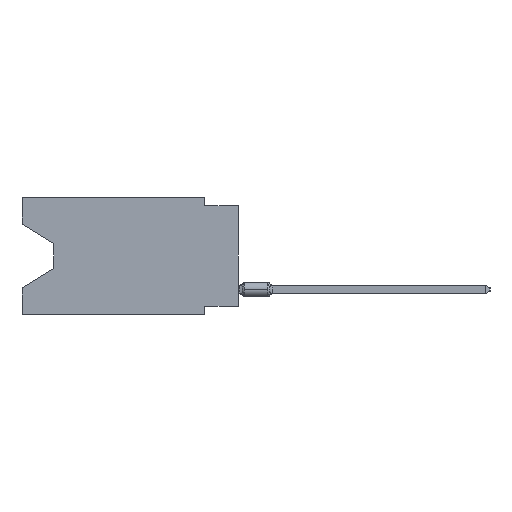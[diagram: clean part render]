
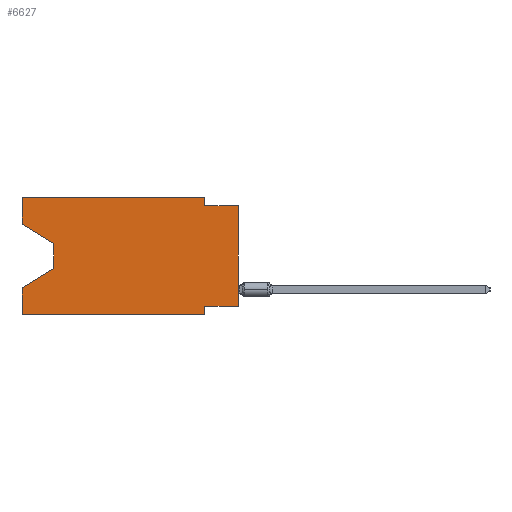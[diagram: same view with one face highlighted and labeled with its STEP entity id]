
A CAD part, left-side view. The second image highlights one B-rep face of the part: STEP entity #6627.
In plain terms, the highlighted planar face has unit normal (-1, 0, 0).
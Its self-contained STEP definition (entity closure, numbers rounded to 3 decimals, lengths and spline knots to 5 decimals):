
#2103 = ORIENTED_EDGE ( 'NONE', *, *, #78197, .T. ) ;
#3496 = DIRECTION ( 'NONE',  ( 1., 0., 0. ) ) ;
#4381 = CARTESIAN_POINT ( 'NONE',  ( 0., 0.645, -0.35 ) ) ;
#5748 = VERTEX_POINT ( 'NONE', #39339 ) ;
#6627 = ADVANCED_FACE ( 'NONE', ( #53965 ), #81701, .F. ) ;
#6694 = CARTESIAN_POINT ( 'NONE',  ( 0., 0.645, -0.08025 ) ) ;
#7017 = LINE ( 'NONE', #53171, #76037 ) ;
#8614 = LINE ( 'NONE', #80415, #32343 ) ;
#9601 = CARTESIAN_POINT ( 'NONE',  ( 0., 0.1, -0.35 ) ) ;
#10518 = LINE ( 'NONE', #36602, #60691 ) ;
#10760 = LINE ( 'NONE', #16331, #52014 ) ;
#13419 = DIRECTION ( 'NONE',  ( 0., -1., 0. ) ) ;
#14014 = CARTESIAN_POINT ( 'NONE',  ( 0., 0.1, -0.025 ) ) ;
#14071 = VERTEX_POINT ( 'NONE', #52846 ) ;
#14917 = ORIENTED_EDGE ( 'NONE', *, *, #15373, .T. ) ;
#15373 = EDGE_CURVE ( 'NONE', #57715, #5748, #27320, .T. ) ;
#16026 = ORIENTED_EDGE ( 'NONE', *, *, #21069, .F. ) ;
#16331 = CARTESIAN_POINT ( 'NONE',  ( 0., 0.645, -0.35 ) ) ;
#17406 = DIRECTION ( 'NONE',  ( 0., -1., 0. ) ) ;
#17515 = CARTESIAN_POINT ( 'NONE',  ( 0., 0.1, -0.325 ) ) ;
#19290 = VECTOR ( 'NONE', #52750, 39.37008 ) ;
#20692 = CARTESIAN_POINT ( 'NONE',  ( 0., 0.55, -0.138 ) ) ;
#20853 = LINE ( 'NONE', #73389, #80168 ) ;
#21069 = EDGE_CURVE ( 'NONE', #24790, #55943, #54844, .T. ) ;
#21274 = DIRECTION ( 'NONE',  ( 0., 0.855, -0.519 ) ) ;
#22059 = CARTESIAN_POINT ( 'NONE',  ( 0., 0.55, -0.212 ) ) ;
#22070 = EDGE_CURVE ( 'NONE', #5748, #50768, #40363, .T. ) ;
#23818 = EDGE_CURVE ( 'NONE', #55943, #52772, #8614, .T. ) ;
#24790 = VERTEX_POINT ( 'NONE', #52839 ) ;
#27320 = LINE ( 'NONE', #32471, #33730 ) ;
#28218 = DIRECTION ( 'NONE',  ( 0., 0., 1. ) ) ;
#28513 = EDGE_LOOP ( 'NONE', ( #14917, #45148, #2103, #65561, #53825, #31459, #16026, #76082, #71676, #73343, #55802, #71684 ) ) ;
#28610 = VECTOR ( 'NONE', #78350, 39.37008 ) ;
#29131 = VERTEX_POINT ( 'NONE', #48868 ) ;
#31459 = ORIENTED_EDGE ( 'NONE', *, *, #23818, .F. ) ;
#32343 = VECTOR ( 'NONE', #62024, 39.37008 ) ;
#32471 = CARTESIAN_POINT ( 'NONE',  ( 0., 0.645, -0.08025 ) ) ;
#33084 = LINE ( 'NONE', #63135, #77907 ) ;
#33103 = VERTEX_POINT ( 'NONE', #65153 ) ;
#33655 = VECTOR ( 'NONE', #28218, 39.37008 ) ;
#33730 = VECTOR ( 'NONE', #40172, 39.37008 ) ;
#34039 = EDGE_CURVE ( 'NONE', #57715, #33103, #10518, .T. ) ;
#36602 = CARTESIAN_POINT ( 'NONE',  ( 0., 0.645, 0. ) ) ;
#38960 = CARTESIAN_POINT ( 'NONE',  ( 0., 0.645, 0. ) ) ;
#39339 = CARTESIAN_POINT ( 'NONE',  ( 0., 0.55, -0.138 ) ) ;
#40172 = DIRECTION ( 'NONE',  ( 0., -0.855, -0.519 ) ) ;
#40363 = LINE ( 'NONE', #20692, #19290 ) ;
#41060 = CARTESIAN_POINT ( 'NONE',  ( 0., 0., 0. ) ) ;
#45039 = CARTESIAN_POINT ( 'NONE',  ( 0., 0.1, 0. ) ) ;
#45148 = ORIENTED_EDGE ( 'NONE', *, *, #22070, .T. ) ;
#48402 = CARTESIAN_POINT ( 'NONE',  ( 0., 0.645, 0. ) ) ;
#48543 = EDGE_CURVE ( 'NONE', #49556, #78808, #78258, .T. ) ;
#48823 = DIRECTION ( 'NONE',  ( 0., -1., 0. ) ) ;
#48868 = CARTESIAN_POINT ( 'NONE',  ( 0., 0., -0.025 ) ) ;
#49556 = VERTEX_POINT ( 'NONE', #4381 ) ;
#50768 = VERTEX_POINT ( 'NONE', #22059 ) ;
#51863 = LINE ( 'NONE', #45039, #28610 ) ;
#51943 = VECTOR ( 'NONE', #66807, 39.37008 ) ;
#52014 = VECTOR ( 'NONE', #48823, 39.37008 ) ;
#52750 = DIRECTION ( 'NONE',  ( 0., 0., -1. ) ) ;
#52772 = VERTEX_POINT ( 'NONE', #9601 ) ;
#52839 = CARTESIAN_POINT ( 'NONE',  ( 0., 0., -0.325 ) ) ;
#52846 = CARTESIAN_POINT ( 'NONE',  ( 0., 0.1, 0. ) ) ;
#53081 = EDGE_CURVE ( 'NONE', #49556, #52772, #10760, .T. ) ;
#53171 = CARTESIAN_POINT ( 'NONE',  ( 0., 0.645, 0. ) ) ;
#53825 = ORIENTED_EDGE ( 'NONE', *, *, #53081, .T. ) ;
#53965 = FACE_OUTER_BOUND ( 'NONE', #28513, .T. ) ;
#54492 = AXIS2_PLACEMENT_3D ( 'NONE', #48402, #3496, #68447 ) ;
#54844 = LINE ( 'NONE', #61664, #51943 ) ;
#55802 = ORIENTED_EDGE ( 'NONE', *, *, #67123, .F. ) ;
#55943 = VERTEX_POINT ( 'NONE', #17515 ) ;
#57715 = VERTEX_POINT ( 'NONE', #6694 ) ;
#59517 = VECTOR ( 'NONE', #79102, 39.37008 ) ;
#60691 = VECTOR ( 'NONE', #62659, 39.37008 ) ;
#60904 = EDGE_CURVE ( 'NONE', #24790, #29131, #73504, .T. ) ;
#61664 = CARTESIAN_POINT ( 'NONE',  ( 0., 0., -0.325 ) ) ;
#62024 = DIRECTION ( 'NONE',  ( 0., 0., -1. ) ) ;
#62659 = DIRECTION ( 'NONE',  ( 0., 0., 1. ) ) ;
#62898 = CARTESIAN_POINT ( 'NONE',  ( 0., 0.645, -0.26975 ) ) ;
#63135 = CARTESIAN_POINT ( 'NONE',  ( 0., 0., -0.025 ) ) ;
#65153 = CARTESIAN_POINT ( 'NONE',  ( 0., 0.645, 0. ) ) ;
#65561 = ORIENTED_EDGE ( 'NONE', *, *, #48543, .F. ) ;
#66807 = DIRECTION ( 'NONE',  ( 0., 1., 0. ) ) ;
#67123 = EDGE_CURVE ( 'NONE', #33103, #14071, #7017, .T. ) ;
#68447 = DIRECTION ( 'NONE',  ( 0., 0., -1. ) ) ;
#68518 = VERTEX_POINT ( 'NONE', #14014 ) ;
#71676 = ORIENTED_EDGE ( 'NONE', *, *, #74771, .F. ) ;
#71684 = ORIENTED_EDGE ( 'NONE', *, *, #34039, .F. ) ;
#73343 = ORIENTED_EDGE ( 'NONE', *, *, #82333, .F. ) ;
#73389 = CARTESIAN_POINT ( 'NONE',  ( 0., 0.55, -0.212 ) ) ;
#73504 = LINE ( 'NONE', #41060, #33655 ) ;
#74771 = EDGE_CURVE ( 'NONE', #68518, #29131, #33084, .T. ) ;
#76037 = VECTOR ( 'NONE', #13419, 39.37008 ) ;
#76082 = ORIENTED_EDGE ( 'NONE', *, *, #60904, .T. ) ;
#77907 = VECTOR ( 'NONE', #17406, 39.37008 ) ;
#78197 = EDGE_CURVE ( 'NONE', #50768, #78808, #20853, .T. ) ;
#78258 = LINE ( 'NONE', #38960, #59517 ) ;
#78350 = DIRECTION ( 'NONE',  ( 0., 0., -1. ) ) ;
#78808 = VERTEX_POINT ( 'NONE', #62898 ) ;
#79102 = DIRECTION ( 'NONE',  ( 0., 0., 1. ) ) ;
#80168 = VECTOR ( 'NONE', #21274, 39.37008 ) ;
#80415 = CARTESIAN_POINT ( 'NONE',  ( 0., 0.1, -0.35 ) ) ;
#81701 = PLANE ( 'NONE',  #54492 ) ;
#82333 = EDGE_CURVE ( 'NONE', #14071, #68518, #51863, .T. ) ;
